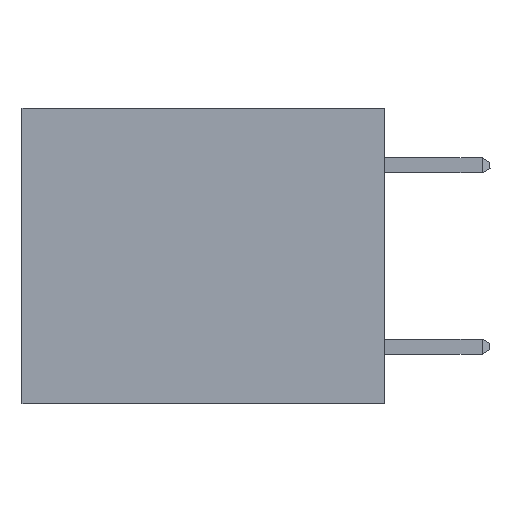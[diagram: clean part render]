
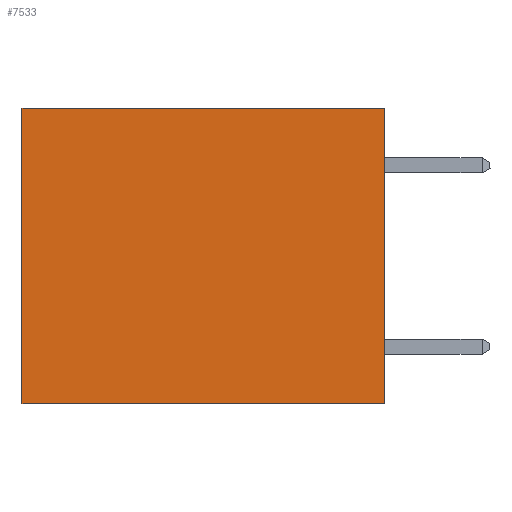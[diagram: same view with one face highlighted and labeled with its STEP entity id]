
A CAD part, left-side view. The second image highlights one B-rep face of the part: STEP entity #7533.
In plain terms, the highlighted planar face has unit normal (-1, 0, 0).
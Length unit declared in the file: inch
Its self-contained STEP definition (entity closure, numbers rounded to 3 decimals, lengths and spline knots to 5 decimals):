
#48 = FACE_OUTER_BOUND ( 'NONE', #8872, .T. ) ;
#2107 = VERTEX_POINT ( 'NONE', #3807 ) ;
#2936 = VECTOR ( 'NONE', #20697, 39.37008 ) ;
#3363 = CARTESIAN_POINT ( 'NONE',  ( 0.3165, 0., -0.49 ) ) ;
#3476 = CARTESIAN_POINT ( 'NONE',  ( 0.3165, 0., -0.49 ) ) ;
#3731 = VERTEX_POINT ( 'NONE', #14466 ) ;
#3807 = CARTESIAN_POINT ( 'NONE',  ( 0.3165, 0.6, -0.49 ) ) ;
#4783 = CARTESIAN_POINT ( 'NONE',  ( 0.3165, 0., 0. ) ) ;
#5447 = ORIENTED_EDGE ( 'NONE', *, *, #17909, .T. ) ;
#5599 = DIRECTION ( 'NONE',  ( 0., 0., -1. ) ) ;
#5642 = CARTESIAN_POINT ( 'NONE',  ( 0.3165, 0.6, -0.49 ) ) ;
#6274 = EDGE_CURVE ( 'NONE', #3731, #2107, #11606, .T. ) ;
#6902 = VERTEX_POINT ( 'NONE', #10818 ) ;
#6939 = DIRECTION ( 'NONE',  ( 0., 1., 0. ) ) ;
#7418 = VERTEX_POINT ( 'NONE', #4783 ) ;
#7533 = ADVANCED_FACE ( 'NONE', ( #48 ), #15630, .F. ) ;
#8872 = EDGE_LOOP ( 'NONE', ( #8947, #21552, #15066, #5447 ) ) ;
#8947 = ORIENTED_EDGE ( 'NONE', *, *, #17507, .T. ) ;
#10557 = DIRECTION ( 'NONE',  ( 1., 0., 0. ) ) ;
#10818 = CARTESIAN_POINT ( 'NONE',  ( 0.3165, 0.6, 0. ) ) ;
#11136 = VECTOR ( 'NONE', #18364, 39.37008 ) ;
#11606 = LINE ( 'NONE', #3476, #13539 ) ;
#12297 = CARTESIAN_POINT ( 'NONE',  ( 0.3165, 0., -0.49 ) ) ;
#12384 = AXIS2_PLACEMENT_3D ( 'NONE', #12297, #10557, #5599 ) ;
#13539 = VECTOR ( 'NONE', #6939, 39.37008 ) ;
#14191 = VECTOR ( 'NONE', #21506, 39.37008 ) ;
#14466 = CARTESIAN_POINT ( 'NONE',  ( 0.3165, 0., -0.49 ) ) ;
#15066 = ORIENTED_EDGE ( 'NONE', *, *, #15928, .F. ) ;
#15630 = PLANE ( 'NONE',  #12384 ) ;
#15928 = EDGE_CURVE ( 'NONE', #7418, #3731, #17688, .T. ) ;
#17507 = EDGE_CURVE ( 'NONE', #6902, #2107, #18115, .T. ) ;
#17688 = LINE ( 'NONE', #3363, #11136 ) ;
#17909 = EDGE_CURVE ( 'NONE', #7418, #6902, #18093, .T. ) ;
#18093 = LINE ( 'NONE', #19662, #14191 ) ;
#18115 = LINE ( 'NONE', #5642, #2936 ) ;
#18364 = DIRECTION ( 'NONE',  ( 0., 0., -1. ) ) ;
#19662 = CARTESIAN_POINT ( 'NONE',  ( 0.3165, 0., 0. ) ) ;
#20697 = DIRECTION ( 'NONE',  ( 0., 0., -1. ) ) ;
#21506 = DIRECTION ( 'NONE',  ( 0., 1., 0. ) ) ;
#21552 = ORIENTED_EDGE ( 'NONE', *, *, #6274, .F. ) ;
